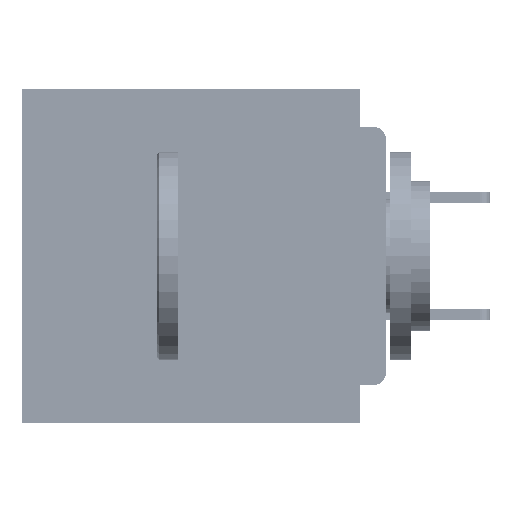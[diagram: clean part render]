
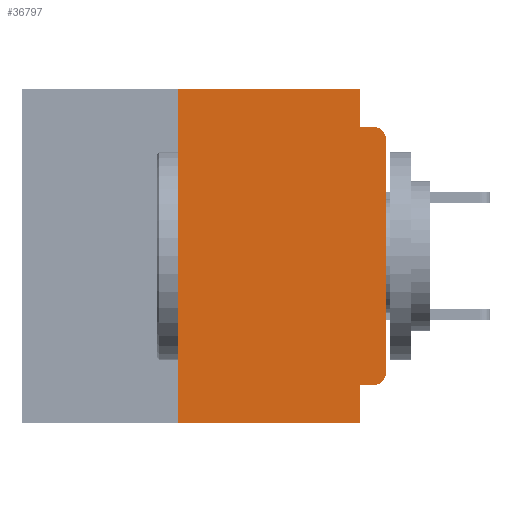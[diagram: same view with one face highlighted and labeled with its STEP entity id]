
A CAD part, left-side view. The second image highlights one B-rep face of the part: STEP entity #36797.
In plain terms, the highlighted planar face has unit normal (-1, 0, 0).
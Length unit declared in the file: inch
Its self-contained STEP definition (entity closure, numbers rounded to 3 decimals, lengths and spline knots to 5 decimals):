
#267 = DIRECTION ( 'NONE',  ( 0., 0., -1. ) ) ;
#503 = AXIS2_PLACEMENT_3D ( 'NONE', #64183, #32254, #267 ) ;
#1195 = VECTOR ( 'NONE', #67193, 39.37008 ) ;
#1358 = CIRCLE ( 'NONE', #62323, 0.015 ) ;
#4068 = DIRECTION ( 'NONE',  ( 0., -1., 0. ) ) ;
#4736 = VECTOR ( 'NONE', #63503, 39.37008 ) ;
#5346 = FACE_OUTER_BOUND ( 'NONE', #25020, .T. ) ;
#6123 = LINE ( 'NONE', #37504, #32870 ) ;
#7260 = VERTEX_POINT ( 'NONE', #8862 ) ;
#8295 = ORIENTED_EDGE ( 'NONE', *, *, #68607, .T. ) ;
#8862 = CARTESIAN_POINT ( 'NONE',  ( 0., 0.031, -0.4 ) ) ;
#10862 = LINE ( 'NONE', #42426, #51808 ) ;
#13697 = LINE ( 'NONE', #29897, #1195 ) ;
#14712 = ORIENTED_EDGE ( 'NONE', *, *, #50238, .T. ) ;
#14853 = ORIENTED_EDGE ( 'NONE', *, *, #15585, .T. ) ;
#15585 = EDGE_CURVE ( 'NONE', #33988, #7260, #40767, .T. ) ;
#15824 = DIRECTION ( 'NONE',  ( 0., 0., -1. ) ) ;
#18499 = EDGE_CURVE ( 'NONE', #28954, #19269, #13697, .T. ) ;
#18511 = CARTESIAN_POINT ( 'NONE',  ( 0., 0.031, -0.045 ) ) ;
#18534 = DIRECTION ( 'NONE',  ( 0., -1., 0. ) ) ;
#18956 = LINE ( 'NONE', #26182, #4736 ) ;
#19269 = VERTEX_POINT ( 'NONE', #30273 ) ;
#19325 = DIRECTION ( 'NONE',  ( -1., 0., 0. ) ) ;
#20573 = EDGE_CURVE ( 'NONE', #53636, #65612, #10862, .T. ) ;
#21501 = VECTOR ( 'NONE', #18534, 39.37008 ) ;
#23463 = EDGE_CURVE ( 'NONE', #33988, #50293, #29163, .T. ) ;
#24026 = CARTESIAN_POINT ( 'NONE',  ( 0., 0.437, -0.4 ) ) ;
#24921 = DIRECTION ( 'NONE',  ( 1., 0., 0. ) ) ;
#25020 = EDGE_LOOP ( 'NONE', ( #32539, #8295, #45477, #36068, #37531, #51851, #14853, #33564, #38859, #14712 ) ) ;
#26182 = CARTESIAN_POINT ( 'NONE',  ( 0., 0.031, -0.4 ) ) ;
#26533 = EDGE_CURVE ( 'NONE', #50293, #53636, #53721, .T. ) ;
#28494 = EDGE_CURVE ( 'NONE', #45004, #48009, #6123, .T. ) ;
#28797 = DIRECTION ( 'NONE',  ( 0., 0., 1. ) ) ;
#28954 = VERTEX_POINT ( 'NONE', #52374 ) ;
#29163 = LINE ( 'NONE', #39314, #66700 ) ;
#29897 = CARTESIAN_POINT ( 'NONE',  ( 0., 0., -0.355 ) ) ;
#30273 = CARTESIAN_POINT ( 'NONE',  ( 0., 0.031, -0.355 ) ) ;
#30733 = CARTESIAN_POINT ( 'NONE',  ( 0., 0.437, 0. ) ) ;
#32254 = DIRECTION ( 'NONE',  ( -1., 0., 0. ) ) ;
#32349 = CARTESIAN_POINT ( 'NONE',  ( 0., 0.015, -0.045 ) ) ;
#32539 = ORIENTED_EDGE ( 'NONE', *, *, #28494, .T. ) ;
#32870 = VECTOR ( 'NONE', #42845, 39.37008 ) ;
#33564 = ORIENTED_EDGE ( 'NONE', *, *, #40322, .F. ) ;
#33988 = VERTEX_POINT ( 'NONE', #35795 ) ;
#35795 = CARTESIAN_POINT ( 'NONE',  ( 0., 0.25, -0.4 ) ) ;
#36068 = ORIENTED_EDGE ( 'NONE', *, *, #20573, .F. ) ;
#36314 = AXIS2_PLACEMENT_3D ( 'NONE', #51510, #24921, #62246 ) ;
#36797 = ADVANCED_FACE ( 'NONE', ( #5346 ), #67386, .F. ) ;
#37504 = CARTESIAN_POINT ( 'NONE',  ( 0., 0., 0. ) ) ;
#37531 = ORIENTED_EDGE ( 'NONE', *, *, #26533, .F. ) ;
#37853 = CARTESIAN_POINT ( 'NONE',  ( 0., 0.25, 0. ) ) ;
#38859 = ORIENTED_EDGE ( 'NONE', *, *, #18499, .F. ) ;
#39314 = CARTESIAN_POINT ( 'NONE',  ( 0., 0.25, -0.4 ) ) ;
#40025 = CARTESIAN_POINT ( 'NONE',  ( 0., 0., -0.045 ) ) ;
#40059 = EDGE_CURVE ( 'NONE', #65612, #54300, #62389, .T. ) ;
#40322 = EDGE_CURVE ( 'NONE', #19269, #7260, #18956, .T. ) ;
#40767 = LINE ( 'NONE', #24026, #54953 ) ;
#42426 = CARTESIAN_POINT ( 'NONE',  ( 0., 0.031, 0. ) ) ;
#42845 = DIRECTION ( 'NONE',  ( 0., 0., 1. ) ) ;
#45004 = VERTEX_POINT ( 'NONE', #59312 ) ;
#45477 = ORIENTED_EDGE ( 'NONE', *, *, #40059, .F. ) ;
#48009 = VERTEX_POINT ( 'NONE', #53047 ) ;
#50238 = EDGE_CURVE ( 'NONE', #28954, #45004, #51255, .T. ) ;
#50293 = VERTEX_POINT ( 'NONE', #37853 ) ;
#50385 = VECTOR ( 'NONE', #4068, 39.37008 ) ;
#51255 = CIRCLE ( 'NONE', #503, 0.015 ) ;
#51280 = CARTESIAN_POINT ( 'NONE',  ( 0., 0.015, -0.06 ) ) ;
#51510 = CARTESIAN_POINT ( 'NONE',  ( 0., 0.437, 0. ) ) ;
#51808 = VECTOR ( 'NONE', #15824, 39.37008 ) ;
#51851 = ORIENTED_EDGE ( 'NONE', *, *, #23463, .F. ) ;
#52374 = CARTESIAN_POINT ( 'NONE',  ( 0., 0.015, -0.355 ) ) ;
#52682 = CARTESIAN_POINT ( 'NONE',  ( 0., 0.031, 0. ) ) ;
#53047 = CARTESIAN_POINT ( 'NONE',  ( 0., 0., -0.06 ) ) ;
#53636 = VERTEX_POINT ( 'NONE', #52682 ) ;
#53721 = LINE ( 'NONE', #30733, #50385 ) ;
#54300 = VERTEX_POINT ( 'NONE', #32349 ) ;
#54953 = VECTOR ( 'NONE', #61345, 39.37008 ) ;
#56645 = DIRECTION ( 'NONE',  ( 0., 0., -1. ) ) ;
#59312 = CARTESIAN_POINT ( 'NONE',  ( 0., 0., -0.34 ) ) ;
#61345 = DIRECTION ( 'NONE',  ( 0., -1., 0. ) ) ;
#62246 = DIRECTION ( 'NONE',  ( 0., 0., -1. ) ) ;
#62323 = AXIS2_PLACEMENT_3D ( 'NONE', #51280, #19325, #56645 ) ;
#62389 = LINE ( 'NONE', #40025, #21501 ) ;
#63503 = DIRECTION ( 'NONE',  ( 0., 0., -1. ) ) ;
#64183 = CARTESIAN_POINT ( 'NONE',  ( 0., 0.015, -0.34 ) ) ;
#65612 = VERTEX_POINT ( 'NONE', #18511 ) ;
#66700 = VECTOR ( 'NONE', #28797, 39.37008 ) ;
#67193 = DIRECTION ( 'NONE',  ( 0., 1., 0. ) ) ;
#67386 = PLANE ( 'NONE',  #36314 ) ;
#68607 = EDGE_CURVE ( 'NONE', #48009, #54300, #1358, .T. ) ;
